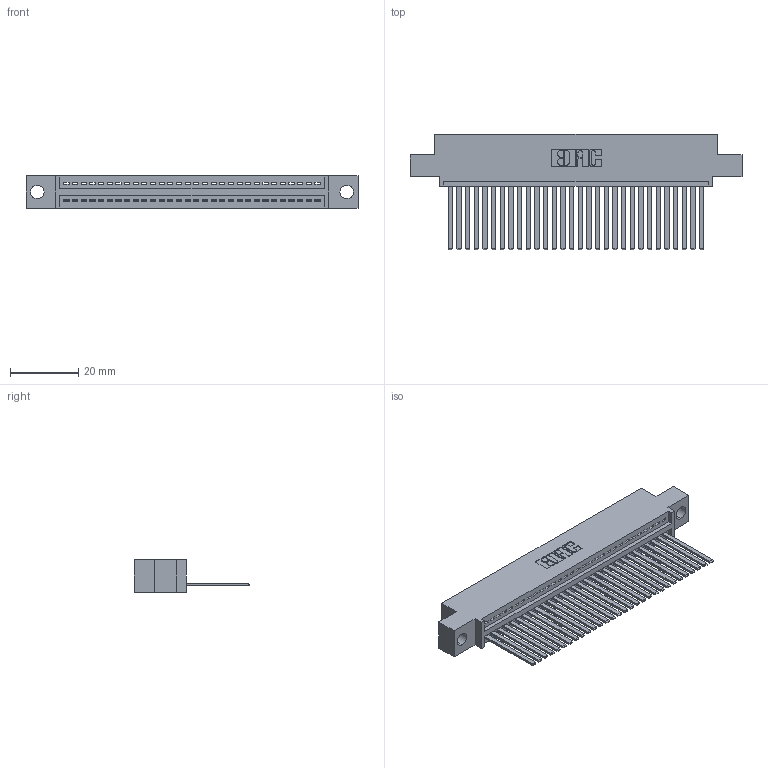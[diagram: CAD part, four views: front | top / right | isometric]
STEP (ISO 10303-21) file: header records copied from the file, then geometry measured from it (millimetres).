
FILE_DESCRIPTION (( 'STEP AP203' ), '1' );
FILE_NAME ('395-030-544-404.STEP', '2021-05-31T14:44:30', ( '' ), ( '' ), 'SwSTEP 2.0', 'SolidWorks 2020', '' );
FILE_SCHEMA (( 'CONFIG_CONTROL_DESIGN' ));
Length unit declared in the file: inch
Products named in the file (3): 345 Part_0.110 Offset - 0.156 Dia-TI; 395-030-544-404; 345-292-001_345-293-144
Assembly tree (31 placements, depth 2):
  395-030-544-404
    345 Part_0.110 Offset - 0.156 Dia-TI
    345-292-001_345-293-144  x30
Bounding box: 97.41 x 33.96 x 9.4 mm (x, y, z)
Volume: 9321.8 mm3; surface area: 13192.2 mm2
Topology: 31 solids, 31 shells, 1704 faces, 5129 edges, 3378 vertices
Faces by surface type: plane 1178, cylinder 526
Entity records: 24561 total; most frequent: CARTESIAN_POINT 4264, ORIENTED_EDGE 4226, DIRECTION 3737, EDGE_CURVE 2113, VECTOR 1865, LINE 1865, VERTEX_POINT 1406, AXIS2_PLACEMENT_3D 936
